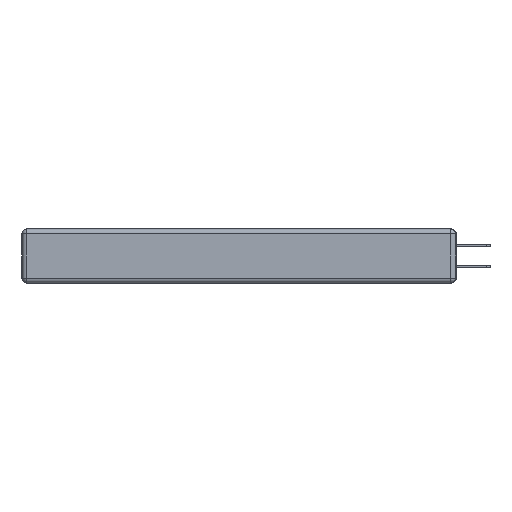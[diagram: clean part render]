
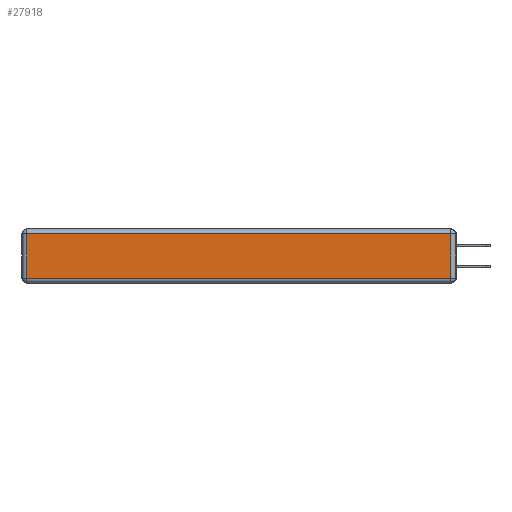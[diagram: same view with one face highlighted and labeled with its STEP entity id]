
A CAD part, left-side view. The second image highlights one B-rep face of the part: STEP entity #27918.
In plain terms, the highlighted planar face has unit normal (-1, 0, 0).
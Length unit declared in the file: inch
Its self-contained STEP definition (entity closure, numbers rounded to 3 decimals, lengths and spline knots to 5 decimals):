
#37 = ORIENTED_EDGE ( 'NONE', *, *, #23445, .T. ) ;
#260 = CARTESIAN_POINT ( 'NONE',  ( 0., 0.03, -0.343 ) ) ;
#815 = CARTESIAN_POINT ( 'NONE',  ( 0., 0.03, -0.313 ) ) ;
#844 = VECTOR ( 'NONE', #4954, 39.37008 ) ;
#2445 = FACE_OUTER_BOUND ( 'NONE', #4618, .T. ) ;
#3483 = EDGE_CURVE ( 'NONE', #18446, #25955, #5709, .T. ) ;
#4618 = EDGE_LOOP ( 'NONE', ( #5453, #37, #24395, #13568 ) ) ;
#4954 = DIRECTION ( 'NONE',  ( 0., 0., 1. ) ) ;
#5305 = DIRECTION ( 'NONE',  ( 0., 1., 0. ) ) ;
#5453 = ORIENTED_EDGE ( 'NONE', *, *, #12488, .T. ) ;
#5709 = LINE ( 'NONE', #17277, #6070 ) ;
#5903 = DIRECTION ( 'NONE',  ( 0., 0., 1. ) ) ;
#6070 = VECTOR ( 'NONE', #27917, 39.37008 ) ;
#6093 = CARTESIAN_POINT ( 'NONE',  ( 0., 0., -0.343 ) ) ;
#6741 = CARTESIAN_POINT ( 'NONE',  ( 0., 2.75, -0.03 ) ) ;
#7004 = AXIS2_PLACEMENT_3D ( 'NONE', #6093, #10668, #5903 ) ;
#7513 = EDGE_CURVE ( 'NONE', #20082, #18446, #13428, .T. ) ;
#8335 = VECTOR ( 'NONE', #5305, 39.37008 ) ;
#10668 = DIRECTION ( 'NONE',  ( -1., 0., 0. ) ) ;
#12488 = EDGE_CURVE ( 'NONE', #25955, #17292, #20225, .T. ) ;
#13428 = LINE ( 'NONE', #6741, #8335 ) ;
#13568 = ORIENTED_EDGE ( 'NONE', *, *, #3483, .T. ) ;
#15191 = CARTESIAN_POINT ( 'NONE',  ( 0., 2.72, -0.03 ) ) ;
#15413 = DIRECTION ( 'NONE',  ( 0., -1., 0. ) ) ;
#17277 = CARTESIAN_POINT ( 'NONE',  ( 0., 2.72, -0.343 ) ) ;
#17292 = VERTEX_POINT ( 'NONE', #815 ) ;
#18446 = VERTEX_POINT ( 'NONE', #15191 ) ;
#18707 = CARTESIAN_POINT ( 'NONE',  ( 0., 2.72, -0.313 ) ) ;
#18862 = VECTOR ( 'NONE', #15413, 39.37008 ) ;
#19645 = CARTESIAN_POINT ( 'NONE',  ( 0., 0., -0.313 ) ) ;
#20082 = VERTEX_POINT ( 'NONE', #26735 ) ;
#20225 = LINE ( 'NONE', #19645, #18862 ) ;
#23154 = LINE ( 'NONE', #260, #844 ) ;
#23445 = EDGE_CURVE ( 'NONE', #17292, #20082, #23154, .T. ) ;
#24395 = ORIENTED_EDGE ( 'NONE', *, *, #7513, .T. ) ;
#25955 = VERTEX_POINT ( 'NONE', #18707 ) ;
#26735 = CARTESIAN_POINT ( 'NONE',  ( 0., 0.03, -0.03 ) ) ;
#27519 = PLANE ( 'NONE',  #7004 ) ;
#27917 = DIRECTION ( 'NONE',  ( 0., 0., -1. ) ) ;
#27918 = ADVANCED_FACE ( 'NONE', ( #2445 ), #27519, .T. ) ;
